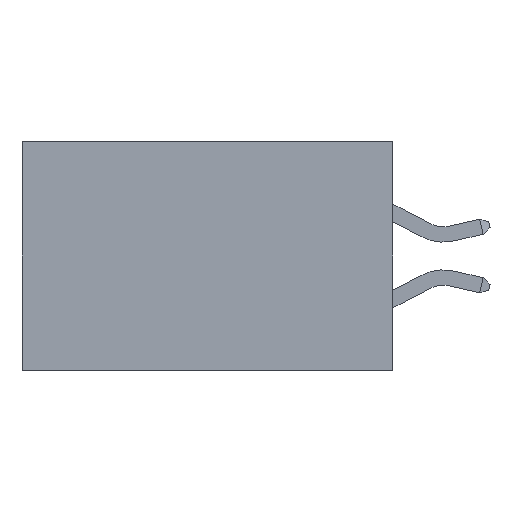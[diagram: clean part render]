
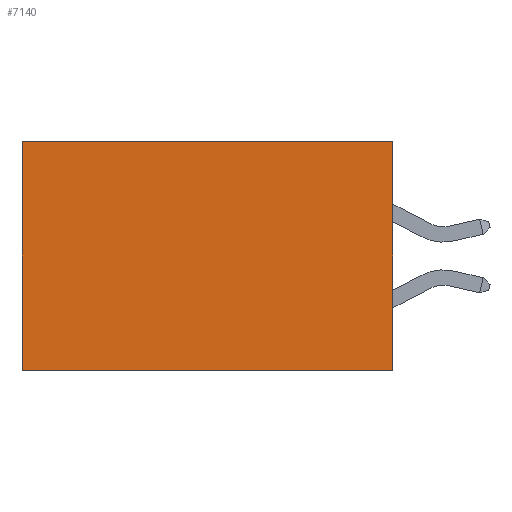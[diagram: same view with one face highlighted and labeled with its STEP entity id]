
A CAD part, left-side view. The second image highlights one B-rep face of the part: STEP entity #7140.
In plain terms, the highlighted planar face has unit normal (-1, 0, 0).
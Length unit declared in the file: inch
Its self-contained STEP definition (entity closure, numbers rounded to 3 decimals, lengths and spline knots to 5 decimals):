
#647 = LINE ( 'NONE', #5525, #10249 ) ;
#820 = EDGE_CURVE ( 'NONE', #7442, #15398, #9614, .T. ) ;
#1816 = EDGE_LOOP ( 'NONE', ( #13877, #2369, #2749, #9668 ) ) ;
#1833 = CARTESIAN_POINT ( 'NONE',  ( 0.2875, 0.6, -0.37 ) ) ;
#2054 = FACE_OUTER_BOUND ( 'NONE', #1816, .T. ) ;
#2222 = CARTESIAN_POINT ( 'NONE',  ( 0.2875, 0.6, 0. ) ) ;
#2369 = ORIENTED_EDGE ( 'NONE', *, *, #13123, .F. ) ;
#2494 = CARTESIAN_POINT ( 'NONE',  ( 0.2875, 0., 0. ) ) ;
#2749 = ORIENTED_EDGE ( 'NONE', *, *, #820, .F. ) ;
#3718 = PLANE ( 'NONE',  #9610 ) ;
#3778 = DIRECTION ( 'NONE',  ( 1., 0., 0. ) ) ;
#4033 = CARTESIAN_POINT ( 'NONE',  ( 0.2875, 0., 0. ) ) ;
#4117 = VECTOR ( 'NONE', #8719, 39.37008 ) ;
#4583 = LINE ( 'NONE', #11496, #7498 ) ;
#5525 = CARTESIAN_POINT ( 'NONE',  ( 0.2875, 0., -0.37 ) ) ;
#6289 = CARTESIAN_POINT ( 'NONE',  ( 0.2875, 0., -0.37 ) ) ;
#6308 = VECTOR ( 'NONE', #11458, 39.37008 ) ;
#6782 = DIRECTION ( 'NONE',  ( 0., 1., 0. ) ) ;
#7140 = ADVANCED_FACE ( 'NONE', ( #2054 ), #3718, .F. ) ;
#7442 = VERTEX_POINT ( 'NONE', #10564 ) ;
#7498 = VECTOR ( 'NONE', #10256, 39.37008 ) ;
#7817 = LINE ( 'NONE', #15928, #4117 ) ;
#8571 = EDGE_CURVE ( 'NONE', #7442, #8930, #4583, .T. ) ;
#8719 = DIRECTION ( 'NONE',  ( 0., 0., -1. ) ) ;
#8930 = VERTEX_POINT ( 'NONE', #2222 ) ;
#9610 = AXIS2_PLACEMENT_3D ( 'NONE', #2494, #3778, #12426 ) ;
#9614 = LINE ( 'NONE', #4033, #6308 ) ;
#9668 = ORIENTED_EDGE ( 'NONE', *, *, #8571, .T. ) ;
#10249 = VECTOR ( 'NONE', #6782, 39.37008 ) ;
#10256 = DIRECTION ( 'NONE',  ( 0., 1., 0. ) ) ;
#10564 = CARTESIAN_POINT ( 'NONE',  ( 0.2875, 0., 0. ) ) ;
#10699 = EDGE_CURVE ( 'NONE', #8930, #15699, #7817, .T. ) ;
#11458 = DIRECTION ( 'NONE',  ( 0., 0., -1. ) ) ;
#11496 = CARTESIAN_POINT ( 'NONE',  ( 0.2875, 0., 0. ) ) ;
#12426 = DIRECTION ( 'NONE',  ( 0., 0., -1. ) ) ;
#13123 = EDGE_CURVE ( 'NONE', #15398, #15699, #647, .T. ) ;
#13877 = ORIENTED_EDGE ( 'NONE', *, *, #10699, .T. ) ;
#15398 = VERTEX_POINT ( 'NONE', #6289 ) ;
#15699 = VERTEX_POINT ( 'NONE', #1833 ) ;
#15928 = CARTESIAN_POINT ( 'NONE',  ( 0.2875, 0.6, 0. ) ) ;
